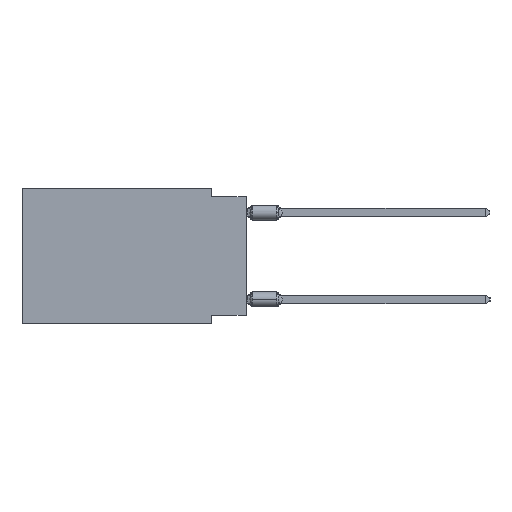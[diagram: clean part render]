
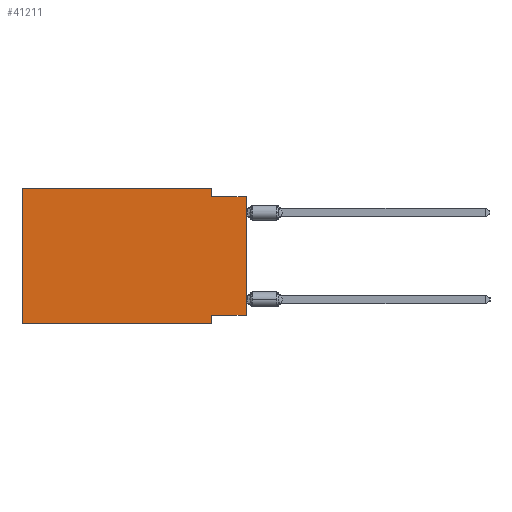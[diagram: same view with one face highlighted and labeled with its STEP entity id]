
A CAD part, left-side view. The second image highlights one B-rep face of the part: STEP entity #41211.
In plain terms, the highlighted planar face has unit normal (-1, 0, 0).
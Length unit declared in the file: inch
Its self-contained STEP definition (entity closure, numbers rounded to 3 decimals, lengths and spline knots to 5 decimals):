
#80 = DIRECTION ( 'NONE',  ( 0., -1., 0. ) ) ;
#360 = LINE ( 'NONE', #41703, #14626 ) ;
#2155 = CARTESIAN_POINT ( 'NONE',  ( 0., 0.645, 0. ) ) ;
#2519 = VECTOR ( 'NONE', #49160, 39.37008 ) ;
#3959 = DIRECTION ( 'NONE',  ( 0., 0., -1. ) ) ;
#4024 = VECTOR ( 'NONE', #52191, 39.37008 ) ;
#4045 = CARTESIAN_POINT ( 'NONE',  ( 0., 0.1, 0. ) ) ;
#4136 = DIRECTION ( 'NONE',  ( 0., -1., 0. ) ) ;
#6474 = LINE ( 'NONE', #31251, #11190 ) ;
#6947 = ORIENTED_EDGE ( 'NONE', *, *, #36557, .F. ) ;
#7104 = CARTESIAN_POINT ( 'NONE',  ( 0., 0.645, 0. ) ) ;
#8039 = CARTESIAN_POINT ( 'NONE',  ( 0., 0.645, -0.39 ) ) ;
#8404 = CARTESIAN_POINT ( 'NONE',  ( 0., 0., 0. ) ) ;
#9334 = ORIENTED_EDGE ( 'NONE', *, *, #42795, .T. ) ;
#11190 = VECTOR ( 'NONE', #3959, 39.37008 ) ;
#12374 = CARTESIAN_POINT ( 'NONE',  ( 0., 0.1, -0.39 ) ) ;
#13152 = CARTESIAN_POINT ( 'NONE',  ( 0., 0.645, 0. ) ) ;
#14343 = VERTEX_POINT ( 'NONE', #7104 ) ;
#14598 = CARTESIAN_POINT ( 'NONE',  ( 0., 0.645, 0. ) ) ;
#14626 = VECTOR ( 'NONE', #80, 39.37008 ) ;
#15778 = PLANE ( 'NONE',  #29936 ) ;
#16950 = ORIENTED_EDGE ( 'NONE', *, *, #19902, .F. ) ;
#18173 = VERTEX_POINT ( 'NONE', #25195 ) ;
#18368 = ORIENTED_EDGE ( 'NONE', *, *, #54000, .T. ) ;
#19389 = DIRECTION ( 'NONE',  ( 1., 0., 0. ) ) ;
#19694 = ORIENTED_EDGE ( 'NONE', *, *, #49935, .F. ) ;
#19902 = EDGE_CURVE ( 'NONE', #20385, #35788, #21910, .T. ) ;
#20361 = VERTEX_POINT ( 'NONE', #4045 ) ;
#20385 = VERTEX_POINT ( 'NONE', #36989 ) ;
#21910 = LINE ( 'NONE', #31187, #42834 ) ;
#24608 = EDGE_CURVE ( 'NONE', #20361, #41756, #6474, .T. ) ;
#25195 = CARTESIAN_POINT ( 'NONE',  ( 0., 0., -0.025 ) ) ;
#25901 = CARTESIAN_POINT ( 'NONE',  ( 0., 0.1, -0.025 ) ) ;
#26882 = VERTEX_POINT ( 'NONE', #40633 ) ;
#27208 = VECTOR ( 'NONE', #4136, 39.37008 ) ;
#29936 = AXIS2_PLACEMENT_3D ( 'NONE', #14598, #19389, #46970 ) ;
#30656 = CARTESIAN_POINT ( 'NONE',  ( 0., 0.645, -0.39 ) ) ;
#30666 = DIRECTION ( 'NONE',  ( 0., 0., -1. ) ) ;
#31135 = LINE ( 'NONE', #13152, #27208 ) ;
#31187 = CARTESIAN_POINT ( 'NONE',  ( 0., 0., -0.365 ) ) ;
#31251 = CARTESIAN_POINT ( 'NONE',  ( 0., 0.1, 0. ) ) ;
#35350 = VERTEX_POINT ( 'NONE', #30656 ) ;
#35600 = LINE ( 'NONE', #8039, #51107 ) ;
#35788 = VERTEX_POINT ( 'NONE', #36221 ) ;
#36221 = CARTESIAN_POINT ( 'NONE',  ( 0., 0.1, -0.365 ) ) ;
#36557 = EDGE_CURVE ( 'NONE', #35788, #26882, #39624, .T. ) ;
#36989 = CARTESIAN_POINT ( 'NONE',  ( 0., 0., -0.365 ) ) ;
#38714 = LINE ( 'NONE', #2155, #4024 ) ;
#39624 = LINE ( 'NONE', #12374, #45035 ) ;
#40296 = EDGE_CURVE ( 'NONE', #35350, #14343, #38714, .T. ) ;
#40633 = CARTESIAN_POINT ( 'NONE',  ( 0., 0.1, -0.39 ) ) ;
#41211 = ADVANCED_FACE ( 'NONE', ( #51454 ), #15778, .F. ) ;
#41703 = CARTESIAN_POINT ( 'NONE',  ( 0., 0., -0.025 ) ) ;
#41756 = VERTEX_POINT ( 'NONE', #25901 ) ;
#42795 = EDGE_CURVE ( 'NONE', #35350, #26882, #35600, .T. ) ;
#42834 = VECTOR ( 'NONE', #58435, 39.37008 ) ;
#45035 = VECTOR ( 'NONE', #30666, 39.37008 ) ;
#45745 = EDGE_LOOP ( 'NONE', ( #18368, #19694, #51551, #48251, #56439, #9334, #6947, #16950 ) ) ;
#46970 = DIRECTION ( 'NONE',  ( 0., 0., -1. ) ) ;
#48251 = ORIENTED_EDGE ( 'NONE', *, *, #51962, .F. ) ;
#48827 = DIRECTION ( 'NONE',  ( 0., -1., 0. ) ) ;
#49160 = DIRECTION ( 'NONE',  ( 0., 0., 1. ) ) ;
#49935 = EDGE_CURVE ( 'NONE', #41756, #18173, #360, .T. ) ;
#51107 = VECTOR ( 'NONE', #48827, 39.37008 ) ;
#51454 = FACE_OUTER_BOUND ( 'NONE', #45745, .T. ) ;
#51551 = ORIENTED_EDGE ( 'NONE', *, *, #24608, .F. ) ;
#51962 = EDGE_CURVE ( 'NONE', #14343, #20361, #31135, .T. ) ;
#52191 = DIRECTION ( 'NONE',  ( 0., 0., 1. ) ) ;
#53366 = LINE ( 'NONE', #8404, #2519 ) ;
#54000 = EDGE_CURVE ( 'NONE', #20385, #18173, #53366, .T. ) ;
#56439 = ORIENTED_EDGE ( 'NONE', *, *, #40296, .F. ) ;
#58435 = DIRECTION ( 'NONE',  ( 0., 1., 0. ) ) ;
